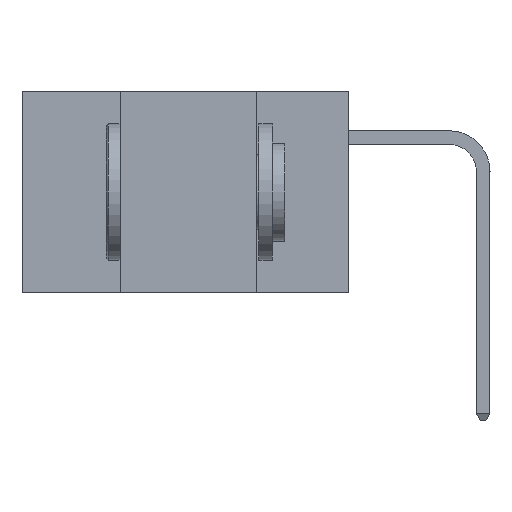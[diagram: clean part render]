
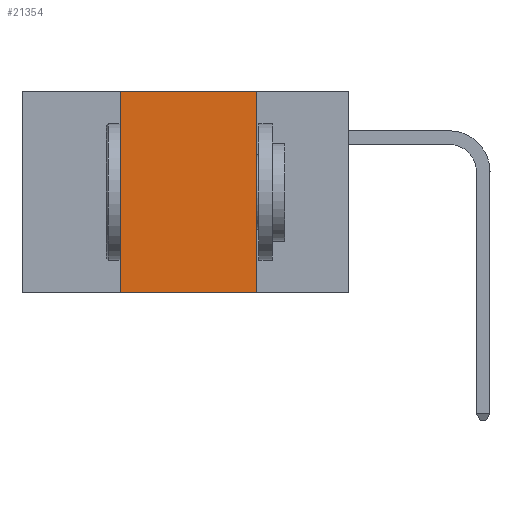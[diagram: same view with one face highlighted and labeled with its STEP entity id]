
A CAD part, left-side view. The second image highlights one B-rep face of the part: STEP entity #21354.
In plain terms, the highlighted planar face has unit normal (-1, 0, 0).
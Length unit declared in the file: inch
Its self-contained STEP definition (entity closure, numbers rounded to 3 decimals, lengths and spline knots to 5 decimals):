
#30 = VECTOR ( 'NONE', #25265, 39.37008 ) ;
#1752 = AXIS2_PLACEMENT_3D ( 'NONE', #3758, #30326, #7629 ) ;
#1786 = DIRECTION ( 'NONE',  ( 0., -1., 0. ) ) ;
#2178 = LINE ( 'NONE', #20114, #21299 ) ;
#2397 = CARTESIAN_POINT ( 'NONE',  ( 0., 0.17, -0.37 ) ) ;
#3463 = ORIENTED_EDGE ( 'NONE', *, *, #33745, .F. ) ;
#3758 = CARTESIAN_POINT ( 'NONE',  ( 0., 0.6, 0. ) ) ;
#7629 = DIRECTION ( 'NONE',  ( 0., 0., -1. ) ) ;
#7718 = VERTEX_POINT ( 'NONE', #36792 ) ;
#7974 = CARTESIAN_POINT ( 'NONE',  ( 0., 0.17, 0. ) ) ;
#8609 = LINE ( 'NONE', #39257, #27602 ) ;
#9108 = LINE ( 'NONE', #47772, #30 ) ;
#9855 = LINE ( 'NONE', #47165, #28845 ) ;
#12757 = VERTEX_POINT ( 'NONE', #38728 ) ;
#13815 = EDGE_CURVE ( 'NONE', #12757, #48624, #9855, .T. ) ;
#16651 = DIRECTION ( 'NONE',  ( 0., 0., -1. ) ) ;
#20114 = CARTESIAN_POINT ( 'NONE',  ( 0., 0.6, 0. ) ) ;
#21299 = VECTOR ( 'NONE', #23940, 39.37008 ) ;
#21354 = ADVANCED_FACE ( 'NONE', ( #42533 ), #49046, .F. ) ;
#23940 = DIRECTION ( 'NONE',  ( 0., -1., 0. ) ) ;
#25265 = DIRECTION ( 'NONE',  ( 0., 0., 1. ) ) ;
#27602 = VECTOR ( 'NONE', #16651, 39.37008 ) ;
#28004 = ORIENTED_EDGE ( 'NONE', *, *, #37900, .F. ) ;
#28845 = VECTOR ( 'NONE', #1786, 39.37008 ) ;
#30326 = DIRECTION ( 'NONE',  ( 1., 0., 0. ) ) ;
#30926 = EDGE_CURVE ( 'NONE', #12757, #7718, #9108, .T. ) ;
#32464 = VERTEX_POINT ( 'NONE', #7974 ) ;
#33635 = ORIENTED_EDGE ( 'NONE', *, *, #30926, .F. ) ;
#33745 = EDGE_CURVE ( 'NONE', #32464, #48624, #8609, .T. ) ;
#36792 = CARTESIAN_POINT ( 'NONE',  ( 0., 0.42, 0. ) ) ;
#37900 = EDGE_CURVE ( 'NONE', #7718, #32464, #2178, .T. ) ;
#38712 = ORIENTED_EDGE ( 'NONE', *, *, #13815, .T. ) ;
#38728 = CARTESIAN_POINT ( 'NONE',  ( 0., 0.42, -0.37 ) ) ;
#39257 = CARTESIAN_POINT ( 'NONE',  ( 0., 0.17, 0. ) ) ;
#42533 = FACE_OUTER_BOUND ( 'NONE', #45422, .T. ) ;
#45422 = EDGE_LOOP ( 'NONE', ( #3463, #28004, #33635, #38712 ) ) ;
#47165 = CARTESIAN_POINT ( 'NONE',  ( 0., 0.6, -0.37 ) ) ;
#47772 = CARTESIAN_POINT ( 'NONE',  ( 0., 0.42, 0. ) ) ;
#48624 = VERTEX_POINT ( 'NONE', #2397 ) ;
#49046 = PLANE ( 'NONE',  #1752 ) ;
